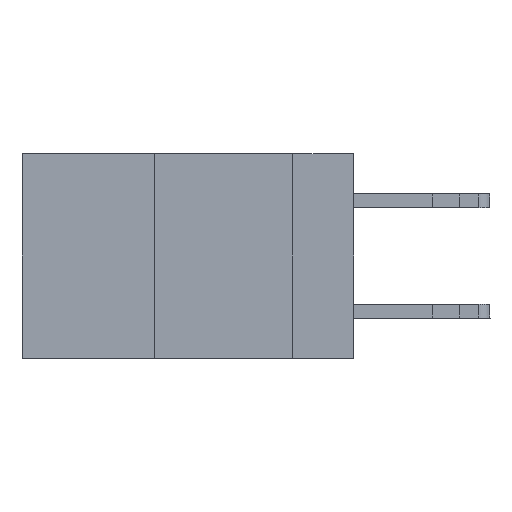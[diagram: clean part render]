
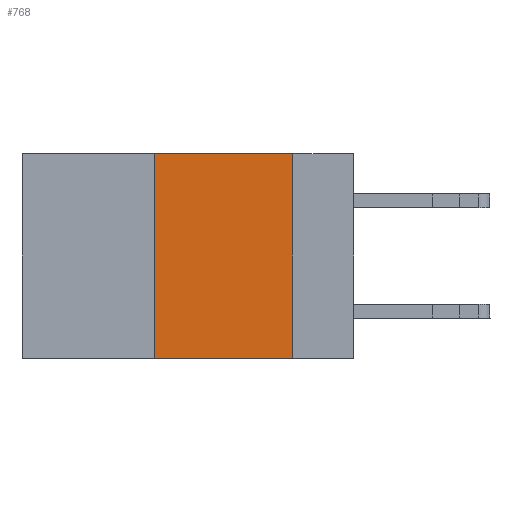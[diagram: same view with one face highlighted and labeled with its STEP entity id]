
A CAD part, left-side view. The second image highlights one B-rep face of the part: STEP entity #768.
In plain terms, the highlighted planar face has unit normal (-1, 0, 0).
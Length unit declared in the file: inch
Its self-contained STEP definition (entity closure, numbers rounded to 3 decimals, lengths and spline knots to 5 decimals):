
#69 = DIRECTION ( 'NONE',  ( 0., -1., 0. ) ) ;
#129 = EDGE_CURVE ( 'NONE', #4283, #1843, #13662, .T. ) ;
#387 = VECTOR ( 'NONE', #4670, 39.37008 ) ;
#607 = VERTEX_POINT ( 'NONE', #5248 ) ;
#768 = ADVANCED_FACE ( 'NONE', ( #5191 ), #15108, .F. ) ;
#1843 = VERTEX_POINT ( 'NONE', #8713 ) ;
#2679 = EDGE_LOOP ( 'NONE', ( #17216, #16927, #16476, #15987 ) ) ;
#4283 = VERTEX_POINT ( 'NONE', #23432 ) ;
#4352 = VERTEX_POINT ( 'NONE', #18382 ) ;
#4670 = DIRECTION ( 'NONE',  ( 0., 0., 1. ) ) ;
#5191 = FACE_OUTER_BOUND ( 'NONE', #2679, .T. ) ;
#5248 = CARTESIAN_POINT ( 'NONE',  ( 0., 0.11, -0.37 ) ) ;
#6971 = CARTESIAN_POINT ( 'NONE',  ( 0., 0.6, 0. ) ) ;
#7015 = DIRECTION ( 'NONE',  ( 1., 0., 0. ) ) ;
#8160 = VECTOR ( 'NONE', #69, 39.37008 ) ;
#8440 = CARTESIAN_POINT ( 'NONE',  ( 0., 0.36, 0. ) ) ;
#8713 = CARTESIAN_POINT ( 'NONE',  ( 0., 0.11, 0. ) ) ;
#9467 = CARTESIAN_POINT ( 'NONE',  ( 0., 0.11, 0. ) ) ;
#12540 = LINE ( 'NONE', #19488, #16755 ) ;
#13662 = LINE ( 'NONE', #6971, #8160 ) ;
#14174 = EDGE_CURVE ( 'NONE', #4352, #607, #12540, .T. ) ;
#14873 = LINE ( 'NONE', #9467, #19644 ) ;
#15108 = PLANE ( 'NONE',  #23596 ) ;
#15811 = LINE ( 'NONE', #8440, #387 ) ;
#15987 = ORIENTED_EDGE ( 'NONE', *, *, #14174, .T. ) ;
#16476 = ORIENTED_EDGE ( 'NONE', *, *, #16594, .F. ) ;
#16594 = EDGE_CURVE ( 'NONE', #4352, #4283, #15811, .T. ) ;
#16683 = DIRECTION ( 'NONE',  ( 0., 0., -1. ) ) ;
#16755 = VECTOR ( 'NONE', #19568, 39.37008 ) ;
#16927 = ORIENTED_EDGE ( 'NONE', *, *, #129, .F. ) ;
#17216 = ORIENTED_EDGE ( 'NONE', *, *, #21421, .F. ) ;
#18382 = CARTESIAN_POINT ( 'NONE',  ( 0., 0.36, -0.37 ) ) ;
#18479 = DIRECTION ( 'NONE',  ( 0., 0., -1. ) ) ;
#18520 = CARTESIAN_POINT ( 'NONE',  ( 0., 0.6, 0. ) ) ;
#19488 = CARTESIAN_POINT ( 'NONE',  ( 0., 0.6, -0.37 ) ) ;
#19568 = DIRECTION ( 'NONE',  ( 0., -1., 0. ) ) ;
#19644 = VECTOR ( 'NONE', #18479, 39.37008 ) ;
#21421 = EDGE_CURVE ( 'NONE', #1843, #607, #14873, .T. ) ;
#23432 = CARTESIAN_POINT ( 'NONE',  ( 0., 0.36, 0. ) ) ;
#23596 = AXIS2_PLACEMENT_3D ( 'NONE', #18520, #7015, #16683 ) ;
